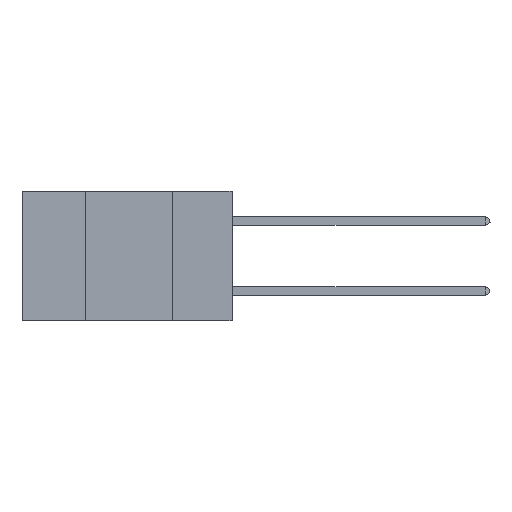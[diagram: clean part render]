
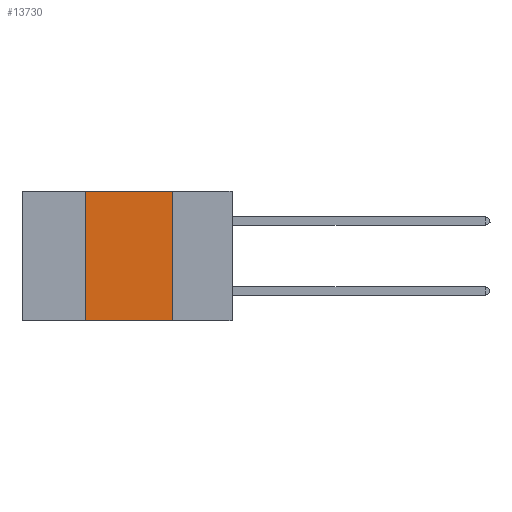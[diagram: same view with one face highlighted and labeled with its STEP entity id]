
A CAD part, left-side view. The second image highlights one B-rep face of the part: STEP entity #13730.
In plain terms, the highlighted planar face has unit normal (-1, 0, 0).
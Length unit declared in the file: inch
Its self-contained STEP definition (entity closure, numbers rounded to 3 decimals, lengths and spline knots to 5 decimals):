
#1801 = VERTEX_POINT ( 'NONE', #5996 ) ;
#2262 = DIRECTION ( 'NONE',  ( 0., -1., 0. ) ) ;
#3276 = LINE ( 'NONE', #4485, #15725 ) ;
#3910 = ORIENTED_EDGE ( 'NONE', *, *, #13548, .F. ) ;
#4485 = CARTESIAN_POINT ( 'NONE',  ( 0., 0.42, 0. ) ) ;
#5996 = CARTESIAN_POINT ( 'NONE',  ( 0., 0.42, -0.37 ) ) ;
#6161 = LINE ( 'NONE', #14155, #19045 ) ;
#6744 = EDGE_CURVE ( 'NONE', #17322, #10045, #9945, .T. ) ;
#7703 = AXIS2_PLACEMENT_3D ( 'NONE', #7829, #19617, #9586 ) ;
#7829 = CARTESIAN_POINT ( 'NONE',  ( 0., 0.6, 0. ) ) ;
#8266 = LINE ( 'NONE', #17721, #21113 ) ;
#9100 = CARTESIAN_POINT ( 'NONE',  ( 0., 0.42, 0. ) ) ;
#9586 = DIRECTION ( 'NONE',  ( 0., 0., -1. ) ) ;
#9945 = LINE ( 'NONE', #18644, #18847 ) ;
#10045 = VERTEX_POINT ( 'NONE', #17730 ) ;
#10403 = FACE_OUTER_BOUND ( 'NONE', #18525, .T. ) ;
#11066 = DIRECTION ( 'NONE',  ( 0., -1., 0. ) ) ;
#11491 = VERTEX_POINT ( 'NONE', #9100 ) ;
#11716 = EDGE_CURVE ( 'NONE', #1801, #11491, #3276, .T. ) ;
#11906 = ORIENTED_EDGE ( 'NONE', *, *, #11716, .F. ) ;
#12956 = EDGE_CURVE ( 'NONE', #1801, #10045, #8266, .T. ) ;
#13548 = EDGE_CURVE ( 'NONE', #11491, #17322, #6161, .T. ) ;
#13730 = ADVANCED_FACE ( 'NONE', ( #10403 ), #17866, .F. ) ;
#14155 = CARTESIAN_POINT ( 'NONE',  ( 0., 0.6, 0. ) ) ;
#14647 = DIRECTION ( 'NONE',  ( 0., 0., 1. ) ) ;
#15725 = VECTOR ( 'NONE', #14647, 39.37008 ) ;
#17322 = VERTEX_POINT ( 'NONE', #19386 ) ;
#17721 = CARTESIAN_POINT ( 'NONE',  ( 0., 0.6, -0.37 ) ) ;
#17730 = CARTESIAN_POINT ( 'NONE',  ( 0., 0.17, -0.37 ) ) ;
#17866 = PLANE ( 'NONE',  #7703 ) ;
#17943 = DIRECTION ( 'NONE',  ( 0., 0., -1. ) ) ;
#18525 = EDGE_LOOP ( 'NONE', ( #20743, #3910, #11906, #20762 ) ) ;
#18644 = CARTESIAN_POINT ( 'NONE',  ( 0., 0.17, 0. ) ) ;
#18847 = VECTOR ( 'NONE', #17943, 39.37008 ) ;
#19045 = VECTOR ( 'NONE', #2262, 39.37008 ) ;
#19386 = CARTESIAN_POINT ( 'NONE',  ( 0., 0.17, 0. ) ) ;
#19617 = DIRECTION ( 'NONE',  ( 1., 0., 0. ) ) ;
#20743 = ORIENTED_EDGE ( 'NONE', *, *, #6744, .F. ) ;
#20762 = ORIENTED_EDGE ( 'NONE', *, *, #12956, .T. ) ;
#21113 = VECTOR ( 'NONE', #11066, 39.37008 ) ;
